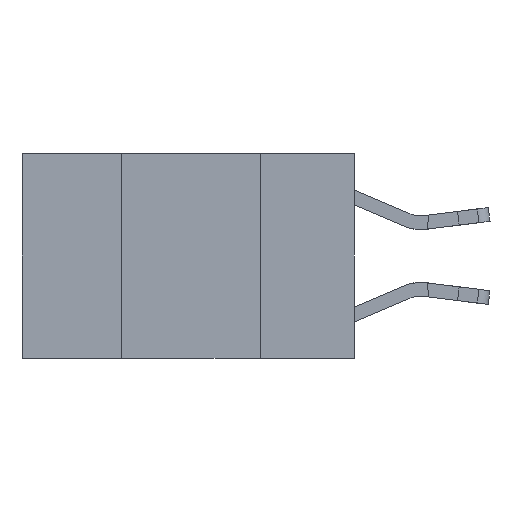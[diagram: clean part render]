
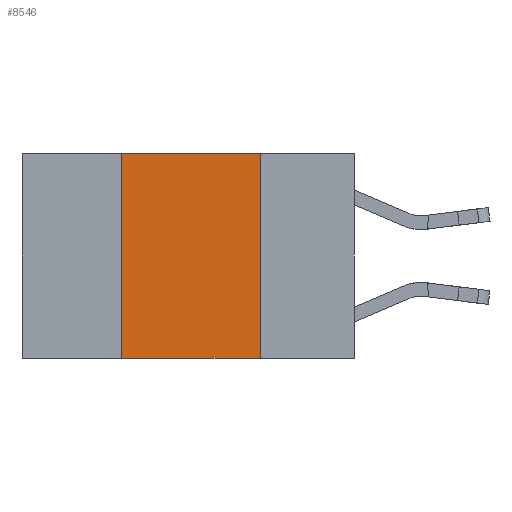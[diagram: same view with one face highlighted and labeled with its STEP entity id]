
A CAD part, left-side view. The second image highlights one B-rep face of the part: STEP entity #8546.
In plain terms, the highlighted planar face has unit normal (-1, 0, 0).
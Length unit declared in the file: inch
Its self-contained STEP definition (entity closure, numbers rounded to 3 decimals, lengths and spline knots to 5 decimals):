
#592 = LINE ( 'NONE', #11837, #14788 ) ;
#678 = DIRECTION ( 'NONE',  ( 1., 0., 0. ) ) ;
#733 = ORIENTED_EDGE ( 'NONE', *, *, #15271, .F. ) ;
#890 = DIRECTION ( 'NONE',  ( 0., -1., 0. ) ) ;
#1241 = CARTESIAN_POINT ( 'NONE',  ( 0., 0.42, 0. ) ) ;
#1279 = AXIS2_PLACEMENT_3D ( 'NONE', #4908, #678, #10430 ) ;
#2820 = FACE_OUTER_BOUND ( 'NONE', #7861, .T. ) ;
#2976 = DIRECTION ( 'NONE',  ( 0., 0., -1. ) ) ;
#3675 = CARTESIAN_POINT ( 'NONE',  ( 0., 0.6, 0. ) ) ;
#3885 = VERTEX_POINT ( 'NONE', #4599 ) ;
#4599 = CARTESIAN_POINT ( 'NONE',  ( 0., 0.42, 0. ) ) ;
#4908 = CARTESIAN_POINT ( 'NONE',  ( 0., 0.6, 0. ) ) ;
#5598 = ORIENTED_EDGE ( 'NONE', *, *, #7961, .F. ) ;
#6929 = CARTESIAN_POINT ( 'NONE',  ( 0., 0.42, -0.37 ) ) ;
#7214 = VERTEX_POINT ( 'NONE', #16971 ) ;
#7282 = VERTEX_POINT ( 'NONE', #13164 ) ;
#7767 = DIRECTION ( 'NONE',  ( 0., -1., 0. ) ) ;
#7861 = EDGE_LOOP ( 'NONE', ( #10188, #5598, #733, #8620 ) ) ;
#7961 = EDGE_CURVE ( 'NONE', #3885, #7282, #14209, .T. ) ;
#8546 = ADVANCED_FACE ( 'NONE', ( #2820 ), #9043, .F. ) ;
#8620 = ORIENTED_EDGE ( 'NONE', *, *, #14392, .T. ) ;
#9043 = PLANE ( 'NONE',  #1279 ) ;
#9290 = VECTOR ( 'NONE', #12299, 39.37008 ) ;
#10110 = VECTOR ( 'NONE', #2976, 39.37008 ) ;
#10188 = ORIENTED_EDGE ( 'NONE', *, *, #16156, .F. ) ;
#10430 = DIRECTION ( 'NONE',  ( 0., 0., -1. ) ) ;
#10545 = LINE ( 'NONE', #16544, #10110 ) ;
#10646 = VECTOR ( 'NONE', #890, 39.37008 ) ;
#11837 = CARTESIAN_POINT ( 'NONE',  ( 0., 0.6, -0.37 ) ) ;
#12299 = DIRECTION ( 'NONE',  ( 0., 0., 1. ) ) ;
#12905 = LINE ( 'NONE', #1241, #9290 ) ;
#13164 = CARTESIAN_POINT ( 'NONE',  ( 0., 0.17, 0. ) ) ;
#14209 = LINE ( 'NONE', #3675, #10646 ) ;
#14392 = EDGE_CURVE ( 'NONE', #14686, #7214, #592, .T. ) ;
#14686 = VERTEX_POINT ( 'NONE', #6929 ) ;
#14788 = VECTOR ( 'NONE', #7767, 39.37008 ) ;
#15271 = EDGE_CURVE ( 'NONE', #14686, #3885, #12905, .T. ) ;
#16156 = EDGE_CURVE ( 'NONE', #7282, #7214, #10545, .T. ) ;
#16544 = CARTESIAN_POINT ( 'NONE',  ( 0., 0.17, 0. ) ) ;
#16971 = CARTESIAN_POINT ( 'NONE',  ( 0., 0.17, -0.37 ) ) ;
